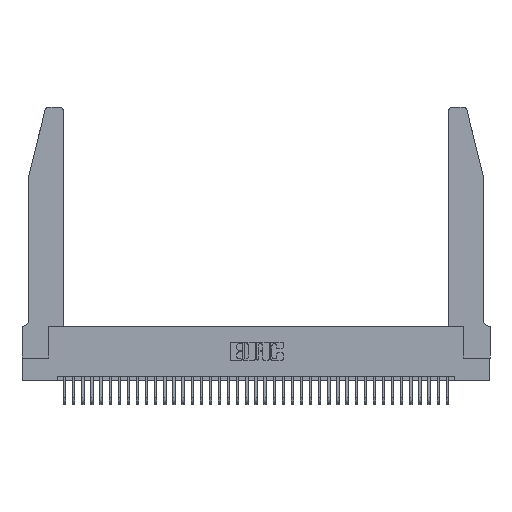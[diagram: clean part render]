
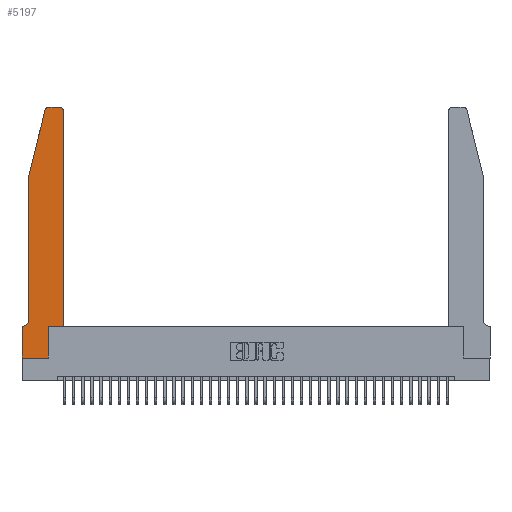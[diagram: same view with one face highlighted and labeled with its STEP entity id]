
A CAD part, top view. The second image highlights one B-rep face of the part: STEP entity #5197.
In plain terms, the highlighted planar face has unit normal (0, 0, 1).
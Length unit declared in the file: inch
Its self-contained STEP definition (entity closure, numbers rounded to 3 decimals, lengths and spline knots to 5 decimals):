
#395 = VERTEX_POINT ( 'NONE', #26238 ) ;
#746 = ORIENTED_EDGE ( 'NONE', *, *, #26054, .T. ) ;
#876 = VECTOR ( 'NONE', #34723, 39.37008 ) ;
#982 = ORIENTED_EDGE ( 'NONE', *, *, #37152, .T. ) ;
#2317 = CARTESIAN_POINT ( 'NONE',  ( 0.0755, 2., 0.37 ) ) ;
#2386 = CARTESIAN_POINT ( 'NONE',  ( 0., 0., 0.37 ) ) ;
#2842 = CARTESIAN_POINT ( 'NONE',  ( 0.284, 2.75, 0.37 ) ) ;
#2908 = ORIENTED_EDGE ( 'NONE', *, *, #35436, .T. ) ;
#4572 = ORIENTED_EDGE ( 'NONE', *, *, #14233, .T. ) ;
#4985 = VERTEX_POINT ( 'NONE', #17624 ) ;
#5197 = ADVANCED_FACE ( 'NONE', ( #14470 ), #23919, .T. ) ;
#5560 = DIRECTION ( 'NONE',  ( 0., -1., 0. ) ) ;
#5878 = AXIS2_PLACEMENT_3D ( 'NONE', #13123, #34422, #16189 ) ;
#6143 = CIRCLE ( 'NONE', #37580, 0.07 ) ;
#6169 = CARTESIAN_POINT ( 'NONE',  ( 0.0755, 0.35, 0.37 ) ) ;
#6518 = VECTOR ( 'NONE', #10218, 39.37008 ) ;
#6632 = LINE ( 'NONE', #19537, #37336 ) ;
#6744 = CARTESIAN_POINT ( 'NONE',  ( 0.0055, 0.42, 0.37 ) ) ;
#7045 = CARTESIAN_POINT ( 'NONE',  ( 0., 0., 0.37 ) ) ;
#7557 = ORIENTED_EDGE ( 'NONE', *, *, #28396, .T. ) ;
#7923 = VECTOR ( 'NONE', #11772, 39.37008 ) ;
#8338 = CARTESIAN_POINT ( 'NONE',  ( 0.2865, 0.35, 0.37 ) ) ;
#8580 = VERTEX_POINT ( 'NONE', #17564 ) ;
#9375 = CARTESIAN_POINT ( 'NONE',  ( 0.25487, 2.72718, 0.37 ) ) ;
#9731 = CARTESIAN_POINT ( 'NONE',  ( 0.284, 2.72, 0.37 ) ) ;
#9862 = DIRECTION ( 'NONE',  ( -1., 0., 0. ) ) ;
#9935 = DIRECTION ( 'NONE',  ( -1., 0., 0. ) ) ;
#10218 = DIRECTION ( 'NONE',  ( 1., 0., 0. ) ) ;
#11202 = CARTESIAN_POINT ( 'NONE',  ( 0.0755, 0.42, 0.37 ) ) ;
#11402 = VECTOR ( 'NONE', #21811, 39.37008 ) ;
#11682 = DIRECTION ( 'NONE',  ( 1., 0., 0. ) ) ;
#11772 = DIRECTION ( 'NONE',  ( 0., 1., 0. ) ) ;
#12888 = DIRECTION ( 'NONE',  ( 1., 0., 0. ) ) ;
#12996 = ORIENTED_EDGE ( 'NONE', *, *, #32214, .T. ) ;
#13071 = CARTESIAN_POINT ( 'NONE',  ( 0.0755, 2., 0.37 ) ) ;
#13123 = CARTESIAN_POINT ( 'NONE',  ( 0.4205, 2.72, 0.37 ) ) ;
#13349 = ORIENTED_EDGE ( 'NONE', *, *, #13592, .T. ) ;
#13592 = EDGE_CURVE ( 'NONE', #30290, #20968, #38122, .T. ) ;
#13872 = VECTOR ( 'NONE', #5560, 39.37008 ) ;
#14233 = EDGE_CURVE ( 'NONE', #395, #37435, #17178, .T. ) ;
#14470 = FACE_OUTER_BOUND ( 'NONE', #20309, .T. ) ;
#14774 = VECTOR ( 'NONE', #9862, 39.37008 ) ;
#14943 = ORIENTED_EDGE ( 'NONE', *, *, #37750, .T. ) ;
#15325 = EDGE_CURVE ( 'NONE', #30195, #30290, #35234, .T. ) ;
#15799 = CARTESIAN_POINT ( 'NONE',  ( 0.2605, 2.75, 0.37 ) ) ;
#16189 = DIRECTION ( 'NONE',  ( 1., 0., 0. ) ) ;
#16318 = CARTESIAN_POINT ( 'NONE',  ( 0.4505, 0.35, 0.37 ) ) ;
#16856 = ORIENTED_EDGE ( 'NONE', *, *, #20705, .T. ) ;
#17178 = LINE ( 'NONE', #36029, #7923 ) ;
#17560 = ORIENTED_EDGE ( 'NONE', *, *, #37662, .T. ) ;
#17564 = CARTESIAN_POINT ( 'NONE',  ( 0.4505, 2.72, 0.37 ) ) ;
#17624 = CARTESIAN_POINT ( 'NONE',  ( 0., 0.35, 0.37 ) ) ;
#17747 = CARTESIAN_POINT ( 'NONE',  ( 0., 0.35, 0.37 ) ) ;
#18172 = CARTESIAN_POINT ( 'NONE',  ( 0.0055, 0.35, 0.37 ) ) ;
#18303 = VERTEX_POINT ( 'NONE', #36893 ) ;
#19537 = CARTESIAN_POINT ( 'NONE',  ( 0.4505, 0.35, 0.37 ) ) ;
#20060 = VECTOR ( 'NONE', #22510, 39.37008 ) ;
#20309 = EDGE_LOOP ( 'NONE', ( #17560, #2908, #28643, #13349, #746, #7557, #982, #34901, #4572, #12996, #14943, #16856 ) ) ;
#20705 = EDGE_CURVE ( 'NONE', #8580, #18303, #23019, .T. ) ;
#20968 = VERTEX_POINT ( 'NONE', #11202 ) ;
#20981 = CARTESIAN_POINT ( 'NONE',  ( 0.0755, 2., 0.37 ) ) ;
#21811 = DIRECTION ( 'NONE',  ( -1., 0., 0. ) ) ;
#22510 = DIRECTION ( 'NONE',  ( 0., 1., 0. ) ) ;
#22616 = DIRECTION ( 'NONE',  ( 1., 0., 0. ) ) ;
#23019 = CIRCLE ( 'NONE', #5878, 0.03 ) ;
#23844 = VERTEX_POINT ( 'NONE', #39702 ) ;
#23919 = PLANE ( 'NONE',  #33088 ) ;
#24056 = DIRECTION ( 'NONE',  ( -0.239, -0.971, 0. ) ) ;
#26054 = EDGE_CURVE ( 'NONE', #20968, #35282, #6143, .T. ) ;
#26238 = CARTESIAN_POINT ( 'NONE',  ( 0.2865, 0., 0.37 ) ) ;
#26785 = LINE ( 'NONE', #28646, #876 ) ;
#27198 = VECTOR ( 'NONE', #24056, 39.37008 ) ;
#28144 = LINE ( 'NONE', #16318, #20060 ) ;
#28339 = DIRECTION ( 'NONE',  ( 0., 0., -1. ) ) ;
#28396 = EDGE_CURVE ( 'NONE', #35282, #4985, #35750, .T. ) ;
#28643 = ORIENTED_EDGE ( 'NONE', *, *, #15325, .T. ) ;
#28646 = CARTESIAN_POINT ( 'NONE',  ( 0., 0., 0.37 ) ) ;
#29989 = DIRECTION ( 'NONE',  ( 0., 0., 1. ) ) ;
#30195 = VERTEX_POINT ( 'NONE', #9375 ) ;
#30290 = VERTEX_POINT ( 'NONE', #13071 ) ;
#31085 = LINE ( 'NONE', #7045, #6518 ) ;
#31161 = DIRECTION ( 'NONE',  ( 0., 0., 1. ) ) ;
#31265 = VERTEX_POINT ( 'NONE', #2842 ) ;
#32214 = EDGE_CURVE ( 'NONE', #37435, #23844, #6632, .T. ) ;
#33088 = AXIS2_PLACEMENT_3D ( 'NONE', #17747, #29989, #11682 ) ;
#33560 = EDGE_CURVE ( 'NONE', #40019, #395, #31085, .T. ) ;
#34202 = AXIS2_PLACEMENT_3D ( 'NONE', #9731, #31161, #12888 ) ;
#34422 = DIRECTION ( 'NONE',  ( 0., 0., 1. ) ) ;
#34723 = DIRECTION ( 'NONE',  ( 0., -1., 0. ) ) ;
#34901 = ORIENTED_EDGE ( 'NONE', *, *, #33560, .T. ) ;
#35234 = LINE ( 'NONE', #20981, #27198 ) ;
#35282 = VERTEX_POINT ( 'NONE', #18172 ) ;
#35436 = EDGE_CURVE ( 'NONE', #31265, #30195, #36771, .T. ) ;
#35750 = LINE ( 'NONE', #6169, #11402 ) ;
#36029 = CARTESIAN_POINT ( 'NONE',  ( 0.2865, 0.35, 0.37 ) ) ;
#36771 = CIRCLE ( 'NONE', #34202, 0.03 ) ;
#36893 = CARTESIAN_POINT ( 'NONE',  ( 0.4205, 2.75, 0.37 ) ) ;
#37152 = EDGE_CURVE ( 'NONE', #4985, #40019, #26785, .T. ) ;
#37336 = VECTOR ( 'NONE', #22616, 39.37008 ) ;
#37435 = VERTEX_POINT ( 'NONE', #8338 ) ;
#37580 = AXIS2_PLACEMENT_3D ( 'NONE', #6744, #28339, #9935 ) ;
#37662 = EDGE_CURVE ( 'NONE', #18303, #31265, #39021, .T. ) ;
#37750 = EDGE_CURVE ( 'NONE', #23844, #8580, #28144, .T. ) ;
#38122 = LINE ( 'NONE', #2317, #13872 ) ;
#39021 = LINE ( 'NONE', #15799, #14774 ) ;
#39702 = CARTESIAN_POINT ( 'NONE',  ( 0.4505, 0.35, 0.37 ) ) ;
#40019 = VERTEX_POINT ( 'NONE', #2386 ) ;
